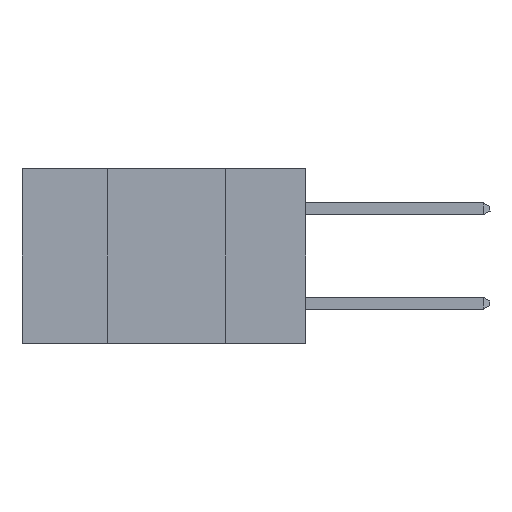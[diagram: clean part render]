
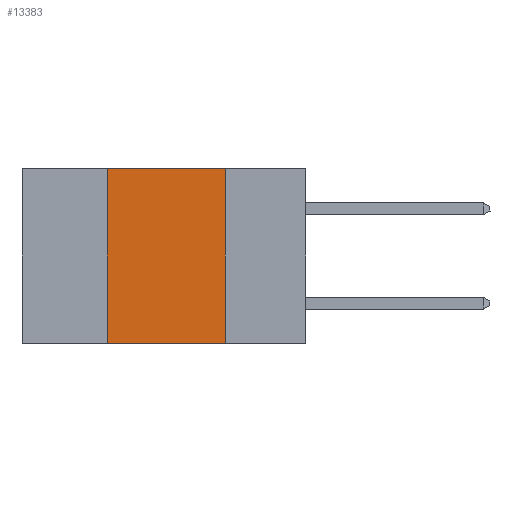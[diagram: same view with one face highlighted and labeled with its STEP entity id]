
A CAD part, left-side view. The second image highlights one B-rep face of the part: STEP entity #13383.
In plain terms, the highlighted planar face has unit normal (-1, 0, 0).
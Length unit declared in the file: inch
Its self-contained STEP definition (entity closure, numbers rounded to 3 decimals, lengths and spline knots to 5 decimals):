
#36 = LINE ( 'NONE', #4074, #5015 ) ;
#190 = VERTEX_POINT ( 'NONE', #2089 ) ;
#246 = VERTEX_POINT ( 'NONE', #477 ) ;
#477 = CARTESIAN_POINT ( 'NONE',  ( 0., 0.42, 0. ) ) ;
#771 = PLANE ( 'NONE',  #3127 ) ;
#1223 = VECTOR ( 'NONE', #2775, 39.37008 ) ;
#1900 = DIRECTION ( 'NONE',  ( 0., -1., 0. ) ) ;
#2089 = CARTESIAN_POINT ( 'NONE',  ( 0., 0.42, -0.37 ) ) ;
#2188 = ORIENTED_EDGE ( 'NONE', *, *, #3163, .F. ) ;
#2775 = DIRECTION ( 'NONE',  ( 0., 0., 1. ) ) ;
#3034 = DIRECTION ( 'NONE',  ( 0., -1., 0. ) ) ;
#3127 = AXIS2_PLACEMENT_3D ( 'NONE', #8607, #4154, #8654 ) ;
#3163 = EDGE_CURVE ( 'NONE', #190, #246, #8312, .T. ) ;
#4074 = CARTESIAN_POINT ( 'NONE',  ( 0., 0.6, 0. ) ) ;
#4154 = DIRECTION ( 'NONE',  ( 1., 0., 0. ) ) ;
#4210 = CARTESIAN_POINT ( 'NONE',  ( 0., 0.6, -0.37 ) ) ;
#4976 = VERTEX_POINT ( 'NONE', #7217 ) ;
#5015 = VECTOR ( 'NONE', #3034, 39.37008 ) ;
#5174 = CARTESIAN_POINT ( 'NONE',  ( 0., 0.42, 0. ) ) ;
#5550 = ORIENTED_EDGE ( 'NONE', *, *, #8634, .F. ) ;
#5631 = EDGE_CURVE ( 'NONE', #190, #4976, #8040, .T. ) ;
#6180 = ORIENTED_EDGE ( 'NONE', *, *, #5631, .T. ) ;
#6201 = DIRECTION ( 'NONE',  ( 0., 0., -1. ) ) ;
#6969 = ORIENTED_EDGE ( 'NONE', *, *, #11559, .F. ) ;
#7208 = VERTEX_POINT ( 'NONE', #13932 ) ;
#7217 = CARTESIAN_POINT ( 'NONE',  ( 0., 0.17, -0.37 ) ) ;
#7824 = EDGE_LOOP ( 'NONE', ( #6969, #5550, #2188, #6180 ) ) ;
#7855 = FACE_OUTER_BOUND ( 'NONE', #7824, .T. ) ;
#8040 = LINE ( 'NONE', #4210, #8393 ) ;
#8312 = LINE ( 'NONE', #5174, #1223 ) ;
#8393 = VECTOR ( 'NONE', #1900, 39.37008 ) ;
#8607 = CARTESIAN_POINT ( 'NONE',  ( 0., 0.6, 0. ) ) ;
#8634 = EDGE_CURVE ( 'NONE', #246, #7208, #36, .T. ) ;
#8654 = DIRECTION ( 'NONE',  ( 0., 0., -1. ) ) ;
#10531 = CARTESIAN_POINT ( 'NONE',  ( 0., 0.17, 0. ) ) ;
#11559 = EDGE_CURVE ( 'NONE', #7208, #4976, #14641, .T. ) ;
#11621 = VECTOR ( 'NONE', #6201, 39.37008 ) ;
#13383 = ADVANCED_FACE ( 'NONE', ( #7855 ), #771, .F. ) ;
#13932 = CARTESIAN_POINT ( 'NONE',  ( 0., 0.17, 0. ) ) ;
#14641 = LINE ( 'NONE', #10531, #11621 ) ;
